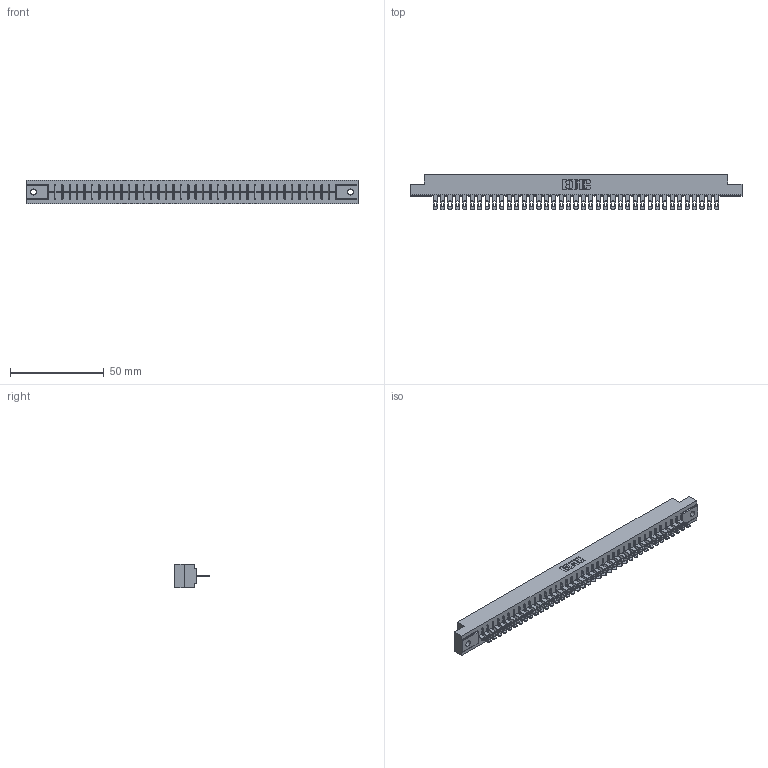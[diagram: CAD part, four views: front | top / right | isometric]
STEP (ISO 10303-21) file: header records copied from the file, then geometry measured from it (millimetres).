
FILE_DESCRIPTION (( 'STEP AP203' ), '1' );
FILE_NAME ('306-039-500-102.STEP', '2019-09-12T00:04:51', ( '' ), ( '' ), 'SwSTEP 2.0', 'SolidWorks 2016', '' );
FILE_SCHEMA (( 'CONFIG_CONTROL_DESIGN' ));
Length unit declared in the file: inch
Products named in the file (3): 306 Part_.128 Dia; 306-290-001_100; 306-039-500-102
Assembly tree (40 placements, depth 2):
  306-039-500-102
    306 Part_.128 Dia
    306-290-001_100  x39
Bounding box: 177.55 x 18.87 x 12.7 mm (x, y, z)
Volume: 19695.5 mm3; surface area: 20596.4 mm2
Topology: 40 solids, 40 shells, 3080 faces, 8701 edges, 5590 vertices
Faces by surface type: plane 2018, cylinder 906, sphere 156
Entity records: 36924 total; most frequent: CARTESIAN_POINT 6200, ORIENTED_EDGE 6146, DIRECTION 6115, EDGE_CURVE 3073, VECTOR 2401, LINE 2401, VERTEX_POINT 1942, AXIS2_PLACEMENT_3D 1857
